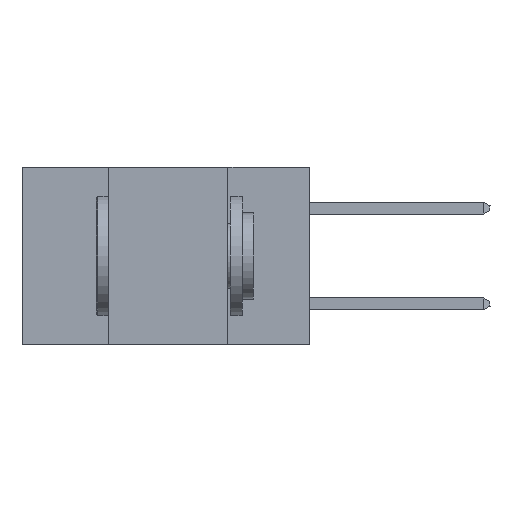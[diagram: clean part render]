
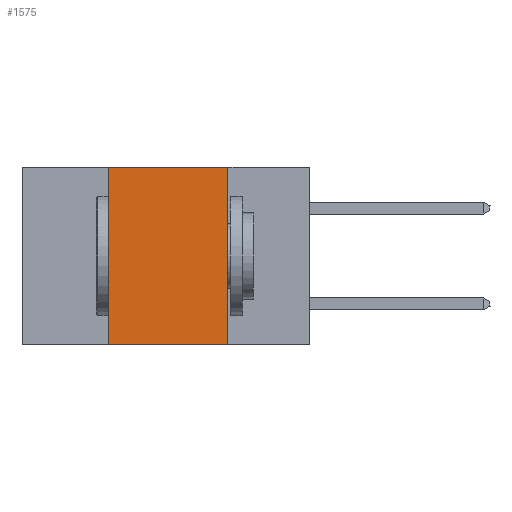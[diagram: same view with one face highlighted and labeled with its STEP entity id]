
A CAD part, left-side view. The second image highlights one B-rep face of the part: STEP entity #1575.
In plain terms, the highlighted planar face has unit normal (-1, 0, 0).
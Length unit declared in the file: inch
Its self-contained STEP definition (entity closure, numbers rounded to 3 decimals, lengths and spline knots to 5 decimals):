
#41 = PLANE ( 'NONE',  #27348 ) ;
#1348 = CARTESIAN_POINT ( 'NONE',  ( 0., 0.17, 0. ) ) ;
#1575 = ADVANCED_FACE ( 'NONE', ( #4850 ), #41, .F. ) ;
#4833 = CARTESIAN_POINT ( 'NONE',  ( 0., 0.6, -0.37 ) ) ;
#4850 = FACE_OUTER_BOUND ( 'NONE', #12472, .T. ) ;
#5326 = LINE ( 'NONE', #4833, #16905 ) ;
#6503 = DIRECTION ( 'NONE',  ( 1., 0., 0. ) ) ;
#8518 = VERTEX_POINT ( 'NONE', #1348 ) ;
#8677 = EDGE_CURVE ( 'NONE', #18124, #8518, #17079, .T. ) ;
#8789 = VERTEX_POINT ( 'NONE', #24449 ) ;
#9275 = VERTEX_POINT ( 'NONE', #26175 ) ;
#9659 = CARTESIAN_POINT ( 'NONE',  ( 0., 0.42, 0. ) ) ;
#12472 = EDGE_LOOP ( 'NONE', ( #20928, #21625, #27500, #22326 ) ) ;
#13232 = DIRECTION ( 'NONE',  ( 0., -1., 0. ) ) ;
#14470 = LINE ( 'NONE', #28365, #25360 ) ;
#15129 = VECTOR ( 'NONE', #24899, 39.37008 ) ;
#15387 = DIRECTION ( 'NONE',  ( 0., 0., -1. ) ) ;
#16403 = VECTOR ( 'NONE', #13232, 39.37008 ) ;
#16905 = VECTOR ( 'NONE', #22273, 39.37008 ) ;
#17079 = LINE ( 'NONE', #21932, #16403 ) ;
#18124 = VERTEX_POINT ( 'NONE', #24396 ) ;
#18751 = CARTESIAN_POINT ( 'NONE',  ( 0., 0.6, 0. ) ) ;
#20928 = ORIENTED_EDGE ( 'NONE', *, *, #28384, .F. ) ;
#21004 = EDGE_CURVE ( 'NONE', #9275, #8789, #5326, .T. ) ;
#21625 = ORIENTED_EDGE ( 'NONE', *, *, #8677, .F. ) ;
#21932 = CARTESIAN_POINT ( 'NONE',  ( 0., 0.6, 0. ) ) ;
#22273 = DIRECTION ( 'NONE',  ( 0., -1., 0. ) ) ;
#22326 = ORIENTED_EDGE ( 'NONE', *, *, #21004, .T. ) ;
#22484 = EDGE_CURVE ( 'NONE', #9275, #18124, #25352, .T. ) ;
#24396 = CARTESIAN_POINT ( 'NONE',  ( 0., 0.42, 0. ) ) ;
#24449 = CARTESIAN_POINT ( 'NONE',  ( 0., 0.17, -0.37 ) ) ;
#24899 = DIRECTION ( 'NONE',  ( 0., 0., 1. ) ) ;
#25352 = LINE ( 'NONE', #9659, #15129 ) ;
#25360 = VECTOR ( 'NONE', #15387, 39.37008 ) ;
#26175 = CARTESIAN_POINT ( 'NONE',  ( 0., 0.42, -0.37 ) ) ;
#27348 = AXIS2_PLACEMENT_3D ( 'NONE', #18751, #6503, #28534 ) ;
#27500 = ORIENTED_EDGE ( 'NONE', *, *, #22484, .F. ) ;
#28365 = CARTESIAN_POINT ( 'NONE',  ( 0., 0.17, 0. ) ) ;
#28384 = EDGE_CURVE ( 'NONE', #8518, #8789, #14470, .T. ) ;
#28534 = DIRECTION ( 'NONE',  ( 0., 0., -1. ) ) ;
